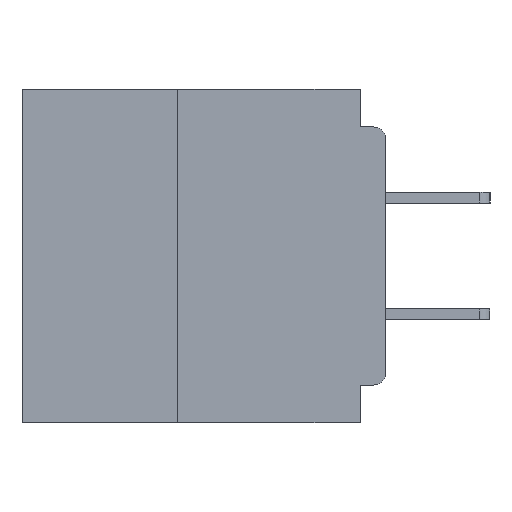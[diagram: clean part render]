
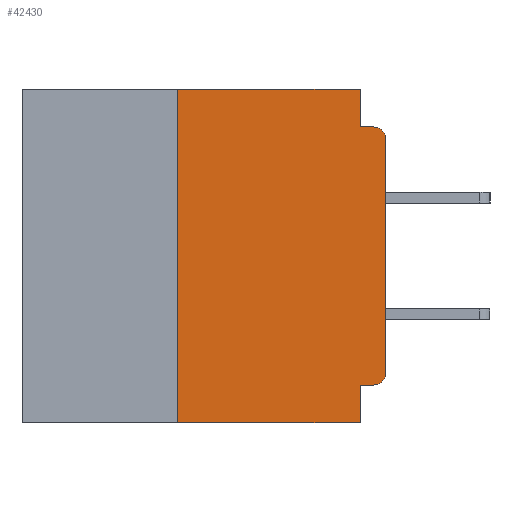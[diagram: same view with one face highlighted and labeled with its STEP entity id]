
A CAD part, left-side view. The second image highlights one B-rep face of the part: STEP entity #42430.
In plain terms, the highlighted planar face has unit normal (-1, 0, 0).
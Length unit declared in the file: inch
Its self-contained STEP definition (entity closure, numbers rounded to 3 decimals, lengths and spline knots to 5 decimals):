
#2242 = CARTESIAN_POINT ( 'NONE',  ( 0., 0., -0.34 ) ) ;
#2481 = DIRECTION ( 'NONE',  ( 0., 0., 1. ) ) ;
#2843 = VERTEX_POINT ( 'NONE', #34076 ) ;
#4477 = VERTEX_POINT ( 'NONE', #43817 ) ;
#5255 = ORIENTED_EDGE ( 'NONE', *, *, #19346, .T. ) ;
#5679 = ORIENTED_EDGE ( 'NONE', *, *, #27464, .T. ) ;
#5894 = DIRECTION ( 'NONE',  ( 1., 0., 0. ) ) ;
#6472 = CARTESIAN_POINT ( 'NONE',  ( 0., 0.25, 0. ) ) ;
#7078 = LINE ( 'NONE', #7652, #16486 ) ;
#7152 = EDGE_CURVE ( 'NONE', #30827, #8223, #36273, .T. ) ;
#7637 = LINE ( 'NONE', #14968, #47739 ) ;
#7652 = CARTESIAN_POINT ( 'NONE',  ( 0., 0.031, 0. ) ) ;
#7997 = VECTOR ( 'NONE', #33829, 39.37008 ) ;
#8050 = CARTESIAN_POINT ( 'NONE',  ( 0., 0.437, 0. ) ) ;
#8223 = VERTEX_POINT ( 'NONE', #32070 ) ;
#9371 = CIRCLE ( 'NONE', #47605, 0.015 ) ;
#10644 = ORIENTED_EDGE ( 'NONE', *, *, #46869, .F. ) ;
#10768 = DIRECTION ( 'NONE',  ( 0., 0., 1. ) ) ;
#11684 = DIRECTION ( 'NONE',  ( 0., 0., -1. ) ) ;
#11879 = CARTESIAN_POINT ( 'NONE',  ( 0., 0.015, -0.34 ) ) ;
#12502 = EDGE_CURVE ( 'NONE', #41026, #8223, #38832, .T. ) ;
#12593 = LINE ( 'NONE', #38910, #32807 ) ;
#12608 = VERTEX_POINT ( 'NONE', #42343 ) ;
#13440 = ORIENTED_EDGE ( 'NONE', *, *, #20643, .F. ) ;
#13788 = EDGE_LOOP ( 'NONE', ( #44646, #5679, #38616, #13440, #10644, #50266, #36266, #34427, #19746, #5255 ) ) ;
#14249 = CARTESIAN_POINT ( 'NONE',  ( 0., 0.015, -0.355 ) ) ;
#14353 = VERTEX_POINT ( 'NONE', #18180 ) ;
#14968 = CARTESIAN_POINT ( 'NONE',  ( 0., 0., -0.355 ) ) ;
#15565 = EDGE_CURVE ( 'NONE', #2843, #4477, #36807, .T. ) ;
#15914 = DIRECTION ( 'NONE',  ( 0., 0., -1. ) ) ;
#16191 = VERTEX_POINT ( 'NONE', #14249 ) ;
#16486 = VECTOR ( 'NONE', #11684, 39.37008 ) ;
#17948 = EDGE_CURVE ( 'NONE', #41026, #36569, #12593, .T. ) ;
#18180 = CARTESIAN_POINT ( 'NONE',  ( 0., 0.031, 0. ) ) ;
#19346 = EDGE_CURVE ( 'NONE', #16191, #38239, #9371, .T. ) ;
#19746 = ORIENTED_EDGE ( 'NONE', *, *, #40837, .F. ) ;
#20643 = EDGE_CURVE ( 'NONE', #14353, #2843, #7078, .T. ) ;
#23281 = DIRECTION ( 'NONE',  ( -1., 0., 0. ) ) ;
#25817 = PLANE ( 'NONE',  #49879 ) ;
#26690 = CARTESIAN_POINT ( 'NONE',  ( 0., 0., 0. ) ) ;
#27391 = LINE ( 'NONE', #8050, #38036 ) ;
#27464 = EDGE_CURVE ( 'NONE', #12608, #4477, #50415, .T. ) ;
#28240 = CARTESIAN_POINT ( 'NONE',  ( 0., 0.25, -0.4 ) ) ;
#30461 = LINE ( 'NONE', #26690, #31758 ) ;
#30561 = AXIS2_PLACEMENT_3D ( 'NONE', #47174, #23281, #51102 ) ;
#30827 = VERTEX_POINT ( 'NONE', #35542 ) ;
#31758 = VECTOR ( 'NONE', #2481, 39.37008 ) ;
#32070 = CARTESIAN_POINT ( 'NONE',  ( 0., 0.031, -0.4 ) ) ;
#32807 = VECTOR ( 'NONE', #10768, 39.37008 ) ;
#33829 = DIRECTION ( 'NONE',  ( 0., -1., 0. ) ) ;
#34062 = DIRECTION ( 'NONE',  ( 0., 0., -1. ) ) ;
#34076 = CARTESIAN_POINT ( 'NONE',  ( 0., 0.031, -0.045 ) ) ;
#34427 = ORIENTED_EDGE ( 'NONE', *, *, #7152, .F. ) ;
#35542 = CARTESIAN_POINT ( 'NONE',  ( 0., 0.031, -0.355 ) ) ;
#36225 = DIRECTION ( 'NONE',  ( 0., -1., 0. ) ) ;
#36266 = ORIENTED_EDGE ( 'NONE', *, *, #12502, .T. ) ;
#36273 = LINE ( 'NONE', #51876, #45552 ) ;
#36569 = VERTEX_POINT ( 'NONE', #6472 ) ;
#36807 = LINE ( 'NONE', #41728, #46103 ) ;
#37200 = EDGE_CURVE ( 'NONE', #38239, #12608, #30461, .T. ) ;
#37736 = DIRECTION ( 'NONE',  ( 0., -1., 0. ) ) ;
#38036 = VECTOR ( 'NONE', #36225, 39.37008 ) ;
#38239 = VERTEX_POINT ( 'NONE', #2242 ) ;
#38616 = ORIENTED_EDGE ( 'NONE', *, *, #15565, .F. ) ;
#38832 = LINE ( 'NONE', #45796, #7997 ) ;
#38910 = CARTESIAN_POINT ( 'NONE',  ( 0., 0.25, -0.4 ) ) ;
#39087 = DIRECTION ( 'NONE',  ( 0., 1., 0. ) ) ;
#40000 = DIRECTION ( 'NONE',  ( -1., 0., 0. ) ) ;
#40837 = EDGE_CURVE ( 'NONE', #16191, #30827, #7637, .T. ) ;
#41026 = VERTEX_POINT ( 'NONE', #28240 ) ;
#41728 = CARTESIAN_POINT ( 'NONE',  ( 0., 0., -0.045 ) ) ;
#42343 = CARTESIAN_POINT ( 'NONE',  ( 0., 0., -0.06 ) ) ;
#42430 = ADVANCED_FACE ( 'NONE', ( #46950 ), #25817, .F. ) ;
#43817 = CARTESIAN_POINT ( 'NONE',  ( 0., 0.015, -0.045 ) ) ;
#44134 = DIRECTION ( 'NONE',  ( 0., 0., -1. ) ) ;
#44646 = ORIENTED_EDGE ( 'NONE', *, *, #37200, .T. ) ;
#45552 = VECTOR ( 'NONE', #44134, 39.37008 ) ;
#45796 = CARTESIAN_POINT ( 'NONE',  ( 0., 0.437, -0.4 ) ) ;
#45868 = CARTESIAN_POINT ( 'NONE',  ( 0., 0.437, 0. ) ) ;
#46103 = VECTOR ( 'NONE', #37736, 39.37008 ) ;
#46869 = EDGE_CURVE ( 'NONE', #36569, #14353, #27391, .T. ) ;
#46950 = FACE_OUTER_BOUND ( 'NONE', #13788, .T. ) ;
#47174 = CARTESIAN_POINT ( 'NONE',  ( 0., 0.015, -0.06 ) ) ;
#47605 = AXIS2_PLACEMENT_3D ( 'NONE', #11879, #40000, #15914 ) ;
#47739 = VECTOR ( 'NONE', #39087, 39.37008 ) ;
#49879 = AXIS2_PLACEMENT_3D ( 'NONE', #45868, #5894, #34062 ) ;
#50266 = ORIENTED_EDGE ( 'NONE', *, *, #17948, .F. ) ;
#50415 = CIRCLE ( 'NONE', #30561, 0.015 ) ;
#51102 = DIRECTION ( 'NONE',  ( 0., 0., -1. ) ) ;
#51876 = CARTESIAN_POINT ( 'NONE',  ( 0., 0.031, -0.4 ) ) ;
